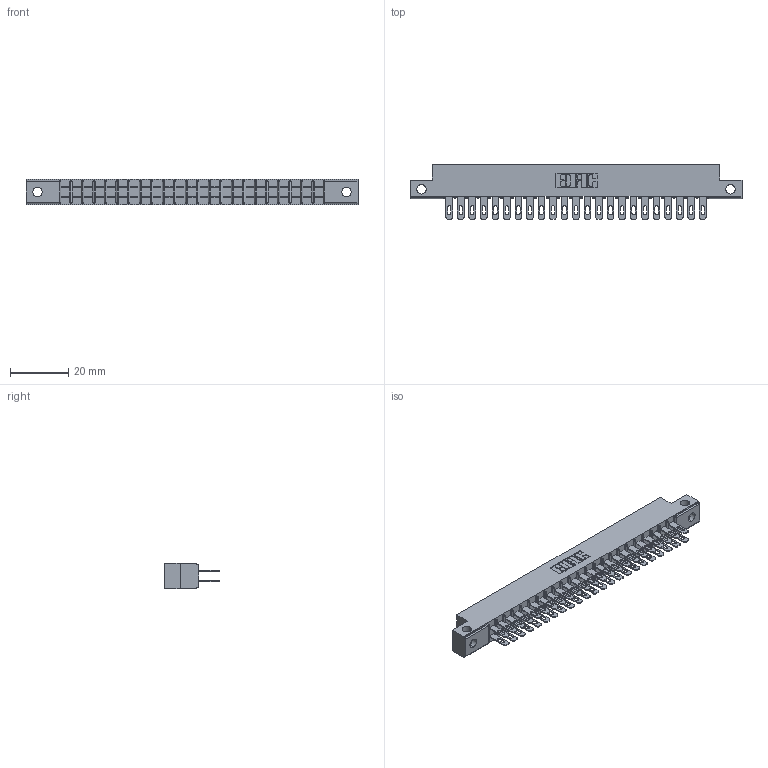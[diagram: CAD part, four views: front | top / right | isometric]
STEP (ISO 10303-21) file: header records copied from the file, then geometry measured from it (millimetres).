
FILE_DESCRIPTION (( 'STEP AP203' ), '1' );
FILE_NAME ('315-046-500-212.STEP', '2020-09-20T02:51:14', ( '' ), ( '' ), 'SwSTEP 2.0', 'SolidWorks 2020', '' );
FILE_SCHEMA (( 'CONFIG_CONTROL_DESIGN' ));
Length unit declared in the file: inch
Products named in the file (3): 305-290-001_500; 305 Part_.128 Dia; 315-046-500-212
Assembly tree (47 placements, depth 2):
  315-046-500-212
    305 Part_.128 Dia
    305-290-001_500  x46
Bounding box: 114.15 x 18.85 x 8.71 mm (x, y, z)
Volume: 7167.9 mm3; surface area: 14390 mm2
Topology: 47 solids, 47 shells, 2428 faces, 6953 edges, 4506 vertices
Faces by surface type: plane 1356, cylinder 980, sphere 92
Entity records: 27644 total; most frequent: CARTESIAN_POINT 4623, ORIENTED_EDGE 4542, DIRECTION 4429, EDGE_CURVE 2271, VECTOR 1797, LINE 1797, VERTEX_POINT 1446, AXIS2_PLACEMENT_3D 1316
